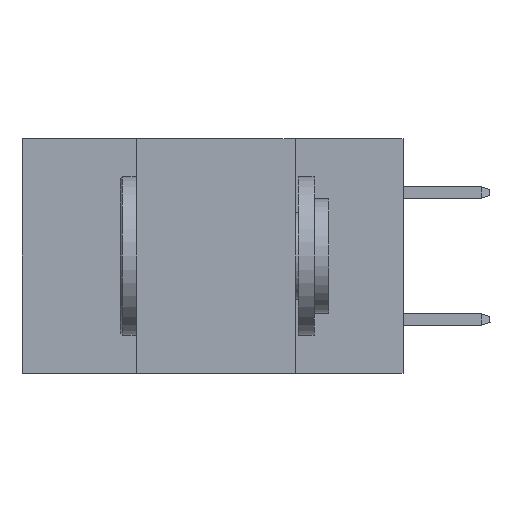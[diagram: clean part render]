
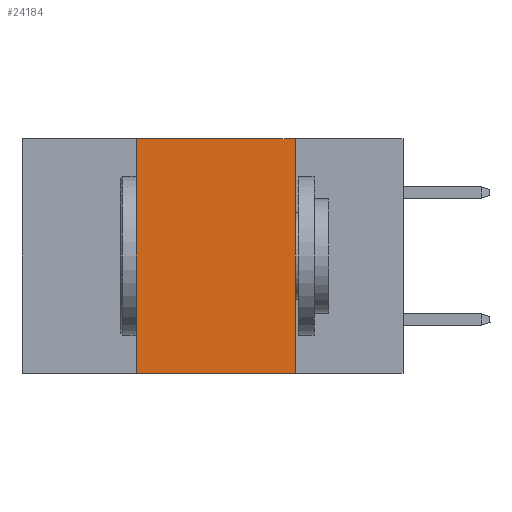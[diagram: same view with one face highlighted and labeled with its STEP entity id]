
A CAD part, left-side view. The second image highlights one B-rep face of the part: STEP entity #24184.
In plain terms, the highlighted planar face has unit normal (-1, 0, 0).
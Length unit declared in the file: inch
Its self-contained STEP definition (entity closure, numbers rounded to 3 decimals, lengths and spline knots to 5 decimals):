
#12 = ORIENTED_EDGE ( 'NONE', *, *, #9325, .F. ) ;
#800 = LINE ( 'NONE', #13288, #17985 ) ;
#2180 = AXIS2_PLACEMENT_3D ( 'NONE', #22234, #20250, #10084 ) ;
#2227 = VERTEX_POINT ( 'NONE', #5210 ) ;
#2776 = CARTESIAN_POINT ( 'NONE',  ( 0., 0.17, 0. ) ) ;
#3274 = EDGE_LOOP ( 'NONE', ( #12, #21349, #24510, #12792 ) ) ;
#4409 = EDGE_CURVE ( 'NONE', #5891, #2227, #22593, .T. ) ;
#4793 = VECTOR ( 'NONE', #18498, 39.37008 ) ;
#5210 = CARTESIAN_POINT ( 'NONE',  ( 0., 0.17, -0.37 ) ) ;
#5891 = VERTEX_POINT ( 'NONE', #15185 ) ;
#9325 = EDGE_CURVE ( 'NONE', #24699, #2227, #20875, .T. ) ;
#10037 = CARTESIAN_POINT ( 'NONE',  ( 0., 0.42, 0. ) ) ;
#10084 = DIRECTION ( 'NONE',  ( 0., 0., -1. ) ) ;
#10573 = EDGE_CURVE ( 'NONE', #14246, #24699, #21059, .T. ) ;
#11158 = CARTESIAN_POINT ( 'NONE',  ( 0., 0.6, 0. ) ) ;
#11200 = DIRECTION ( 'NONE',  ( 0., 0., 1. ) ) ;
#12032 = CARTESIAN_POINT ( 'NONE',  ( 0., 0.6, -0.37 ) ) ;
#12792 = ORIENTED_EDGE ( 'NONE', *, *, #4409, .T. ) ;
#13288 = CARTESIAN_POINT ( 'NONE',  ( 0., 0.42, 0. ) ) ;
#14246 = VERTEX_POINT ( 'NONE', #10037 ) ;
#15185 = CARTESIAN_POINT ( 'NONE',  ( 0., 0.42, -0.37 ) ) ;
#17026 = DIRECTION ( 'NONE',  ( 0., 0., -1. ) ) ;
#17152 = EDGE_CURVE ( 'NONE', #5891, #14246, #800, .T. ) ;
#17985 = VECTOR ( 'NONE', #11200, 39.37008 ) ;
#17998 = FACE_OUTER_BOUND ( 'NONE', #3274, .T. ) ;
#18498 = DIRECTION ( 'NONE',  ( 0., -1., 0. ) ) ;
#20250 = DIRECTION ( 'NONE',  ( 1., 0., 0. ) ) ;
#20875 = LINE ( 'NONE', #2776, #21217 ) ;
#21059 = LINE ( 'NONE', #11158, #24659 ) ;
#21217 = VECTOR ( 'NONE', #17026, 39.37008 ) ;
#21349 = ORIENTED_EDGE ( 'NONE', *, *, #10573, .F. ) ;
#22234 = CARTESIAN_POINT ( 'NONE',  ( 0., 0.6, 0. ) ) ;
#22593 = LINE ( 'NONE', #12032, #4793 ) ;
#23044 = DIRECTION ( 'NONE',  ( 0., -1., 0. ) ) ;
#23908 = CARTESIAN_POINT ( 'NONE',  ( 0., 0.17, 0. ) ) ;
#23937 = PLANE ( 'NONE',  #2180 ) ;
#24184 = ADVANCED_FACE ( 'NONE', ( #17998 ), #23937, .F. ) ;
#24510 = ORIENTED_EDGE ( 'NONE', *, *, #17152, .F. ) ;
#24659 = VECTOR ( 'NONE', #23044, 39.37008 ) ;
#24699 = VERTEX_POINT ( 'NONE', #23908 ) ;
